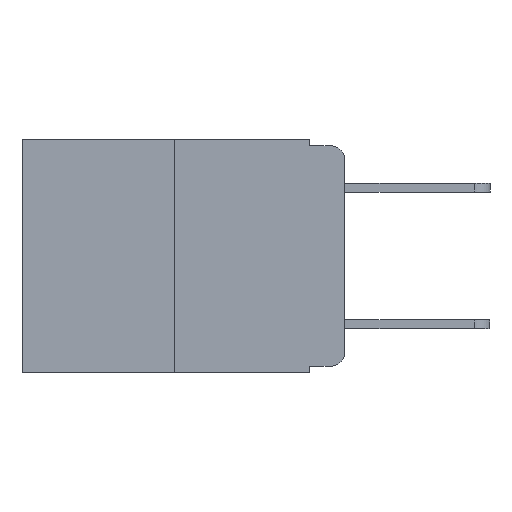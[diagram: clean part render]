
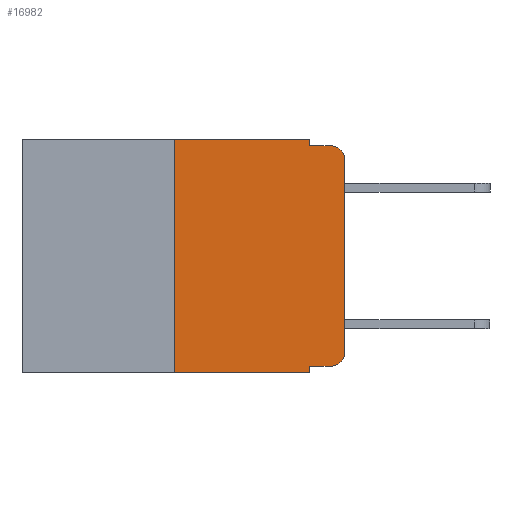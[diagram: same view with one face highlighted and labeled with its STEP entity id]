
A CAD part, left-side view. The second image highlights one B-rep face of the part: STEP entity #16982.
In plain terms, the highlighted planar face has unit normal (-1, 0, 0).
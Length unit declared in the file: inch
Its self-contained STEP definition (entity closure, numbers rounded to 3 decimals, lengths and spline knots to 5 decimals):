
#219 = CARTESIAN_POINT ( 'NONE',  ( 0., 0.051, -0.333 ) ) ;
#1317 = EDGE_CURVE ( 'NONE', #15799, #4773, #6383, .T. ) ;
#1431 = ORIENTED_EDGE ( 'NONE', *, *, #6992, .F. ) ;
#1484 = CARTESIAN_POINT ( 'NONE',  ( 0., 0.051, -0.01 ) ) ;
#1894 = DIRECTION ( 'NONE',  ( 0., 0., 1. ) ) ;
#2009 = DIRECTION ( 'NONE',  ( 0., 0., -1. ) ) ;
#2202 = LINE ( 'NONE', #16694, #15800 ) ;
#2306 = CARTESIAN_POINT ( 'NONE',  ( 0., 0.02, -0.03 ) ) ;
#2404 = CARTESIAN_POINT ( 'NONE',  ( 0., 0.473, 0. ) ) ;
#2706 = ORIENTED_EDGE ( 'NONE', *, *, #20543, .T. ) ;
#2761 = ORIENTED_EDGE ( 'NONE', *, *, #8576, .T. ) ;
#2889 = VERTEX_POINT ( 'NONE', #13730 ) ;
#3038 = EDGE_CURVE ( 'NONE', #8346, #12969, #2202, .T. ) ;
#4028 = ORIENTED_EDGE ( 'NONE', *, *, #20480, .F. ) ;
#4158 = ORIENTED_EDGE ( 'NONE', *, *, #7119, .F. ) ;
#4170 = DIRECTION ( 'NONE',  ( 0., 0., -1. ) ) ;
#4630 = CARTESIAN_POINT ( 'NONE',  ( 0., 0.051, -0.01 ) ) ;
#4773 = VERTEX_POINT ( 'NONE', #16053 ) ;
#4893 = VECTOR ( 'NONE', #11050, 39.37008 ) ;
#4906 = ORIENTED_EDGE ( 'NONE', *, *, #14912, .F. ) ;
#5004 = LINE ( 'NONE', #14447, #21788 ) ;
#5010 = ORIENTED_EDGE ( 'NONE', *, *, #3038, .F. ) ;
#5824 = VECTOR ( 'NONE', #13594, 39.37008 ) ;
#6083 = CARTESIAN_POINT ( 'NONE',  ( 0., 0.02, -0.313 ) ) ;
#6162 = ORIENTED_EDGE ( 'NONE', *, *, #14412, .T. ) ;
#6383 = LINE ( 'NONE', #219, #5824 ) ;
#6415 = LINE ( 'NONE', #4630, #15174 ) ;
#6441 = DIRECTION ( 'NONE',  ( 0., -1., 0. ) ) ;
#6992 = EDGE_CURVE ( 'NONE', #12969, #7490, #12346, .T. ) ;
#7119 = EDGE_CURVE ( 'NONE', #7490, #19103, #18821, .T. ) ;
#7490 = VERTEX_POINT ( 'NONE', #20310 ) ;
#7662 = VECTOR ( 'NONE', #11227, 39.37008 ) ;
#7845 = DIRECTION ( 'NONE',  ( 0., 0., -1. ) ) ;
#8236 = FACE_OUTER_BOUND ( 'NONE', #13225, .T. ) ;
#8284 = CARTESIAN_POINT ( 'NONE',  ( 0., 0.473, -0.343 ) ) ;
#8346 = VERTEX_POINT ( 'NONE', #17516 ) ;
#8494 = VERTEX_POINT ( 'NONE', #14429 ) ;
#8558 = ORIENTED_EDGE ( 'NONE', *, *, #21478, .T. ) ;
#8576 = EDGE_CURVE ( 'NONE', #2889, #8494, #9421, .T. ) ;
#9421 = CIRCLE ( 'NONE', #14558, 0.02 ) ;
#9637 = DIRECTION ( 'NONE',  ( 1., 0., 0. ) ) ;
#9728 = VECTOR ( 'NONE', #12860, 39.37008 ) ;
#11050 = DIRECTION ( 'NONE',  ( 0., 0., -1. ) ) ;
#11098 = CARTESIAN_POINT ( 'NONE',  ( 0., 0., 0. ) ) ;
#11227 = DIRECTION ( 'NONE',  ( 0., -1., 0. ) ) ;
#12346 = LINE ( 'NONE', #18564, #7662 ) ;
#12860 = DIRECTION ( 'NONE',  ( 0., 0., 1. ) ) ;
#12969 = VERTEX_POINT ( 'NONE', #18627 ) ;
#13143 = CARTESIAN_POINT ( 'NONE',  ( 0., 0., -0.313 ) ) ;
#13225 = EDGE_LOOP ( 'NONE', ( #6162, #2761, #4028, #4158, #1431, #5010, #2706, #4906, #20488, #8558 ) ) ;
#13251 = VERTEX_POINT ( 'NONE', #14575 ) ;
#13594 = DIRECTION ( 'NONE',  ( 0., -1., 0. ) ) ;
#13730 = CARTESIAN_POINT ( 'NONE',  ( 0., 0., -0.03 ) ) ;
#14073 = VECTOR ( 'NONE', #22041, 39.37008 ) ;
#14412 = EDGE_CURVE ( 'NONE', #16990, #2889, #18400, .T. ) ;
#14429 = CARTESIAN_POINT ( 'NONE',  ( 0., 0.02, -0.01 ) ) ;
#14447 = CARTESIAN_POINT ( 'NONE',  ( 0., 0.051, 0. ) ) ;
#14558 = AXIS2_PLACEMENT_3D ( 'NONE', #2306, #14725, #4170 ) ;
#14575 = CARTESIAN_POINT ( 'NONE',  ( 0., 0.051, -0.343 ) ) ;
#14725 = DIRECTION ( 'NONE',  ( -1., 0., 0. ) ) ;
#14893 = AXIS2_PLACEMENT_3D ( 'NONE', #6083, #18259, #7845 ) ;
#14912 = EDGE_CURVE ( 'NONE', #15799, #13251, #5004, .T. ) ;
#15174 = VECTOR ( 'NONE', #6441, 39.37008 ) ;
#15799 = VERTEX_POINT ( 'NONE', #21758 ) ;
#15800 = VECTOR ( 'NONE', #1894, 39.37008 ) ;
#16053 = CARTESIAN_POINT ( 'NONE',  ( 0., 0.02, -0.333 ) ) ;
#16694 = CARTESIAN_POINT ( 'NONE',  ( 0., 0.25, 0. ) ) ;
#16982 = ADVANCED_FACE ( 'NONE', ( #8236 ), #18266, .F. ) ;
#16990 = VERTEX_POINT ( 'NONE', #13143 ) ;
#17516 = CARTESIAN_POINT ( 'NONE',  ( 0., 0.25, -0.343 ) ) ;
#17540 = AXIS2_PLACEMENT_3D ( 'NONE', #2404, #9637, #21648 ) ;
#18259 = DIRECTION ( 'NONE',  ( -1., 0., 0. ) ) ;
#18266 = PLANE ( 'NONE',  #17540 ) ;
#18400 = LINE ( 'NONE', #11098, #9728 ) ;
#18564 = CARTESIAN_POINT ( 'NONE',  ( 0., 0.473, 0. ) ) ;
#18627 = CARTESIAN_POINT ( 'NONE',  ( 0., 0.25, 0. ) ) ;
#18649 = LINE ( 'NONE', #8284, #14073 ) ;
#18821 = LINE ( 'NONE', #22007, #4893 ) ;
#19103 = VERTEX_POINT ( 'NONE', #1484 ) ;
#20310 = CARTESIAN_POINT ( 'NONE',  ( 0., 0.051, 0. ) ) ;
#20480 = EDGE_CURVE ( 'NONE', #19103, #8494, #6415, .T. ) ;
#20488 = ORIENTED_EDGE ( 'NONE', *, *, #1317, .T. ) ;
#20543 = EDGE_CURVE ( 'NONE', #8346, #13251, #18649, .T. ) ;
#21478 = EDGE_CURVE ( 'NONE', #4773, #16990, #21488, .T. ) ;
#21488 = CIRCLE ( 'NONE', #14893, 0.02 ) ;
#21648 = DIRECTION ( 'NONE',  ( 0., 0., -1. ) ) ;
#21758 = CARTESIAN_POINT ( 'NONE',  ( 0., 0.051, -0.333 ) ) ;
#21788 = VECTOR ( 'NONE', #2009, 39.37008 ) ;
#22007 = CARTESIAN_POINT ( 'NONE',  ( 0., 0.051, 0. ) ) ;
#22041 = DIRECTION ( 'NONE',  ( 0., -1., 0. ) ) ;
